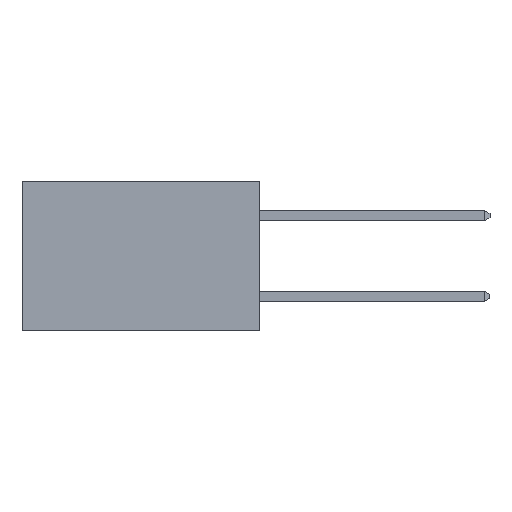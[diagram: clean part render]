
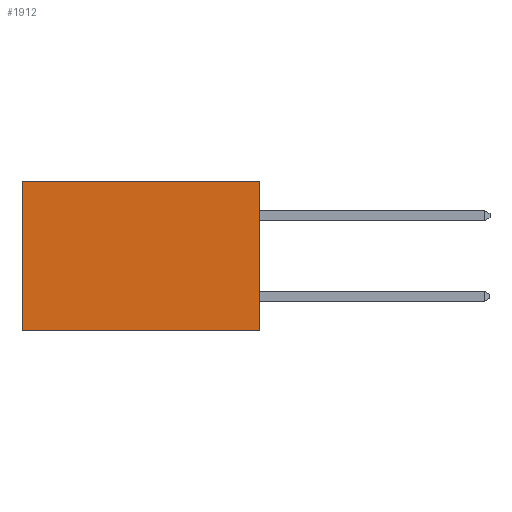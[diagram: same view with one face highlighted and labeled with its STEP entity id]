
A CAD part, left-side view. The second image highlights one B-rep face of the part: STEP entity #1912.
In plain terms, the highlighted planar face has unit normal (-1, 0, 0).
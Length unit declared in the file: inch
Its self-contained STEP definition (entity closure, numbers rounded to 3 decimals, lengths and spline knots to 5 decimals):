
#59 = DIRECTION ( 'NONE',  ( 0., 1., 0. ) ) ;
#163 = DIRECTION ( 'NONE',  ( 0., 1., 0. ) ) ;
#403 = EDGE_LOOP ( 'NONE', ( #11225, #3974, #9107, #4269 ) ) ;
#441 = LINE ( 'NONE', #2921, #5228 ) ;
#537 = EDGE_CURVE ( 'NONE', #11483, #9231, #3000, .T. ) ;
#574 = CARTESIAN_POINT ( 'NONE',  ( 0.277, 0., -0.37 ) ) ;
#1319 = AXIS2_PLACEMENT_3D ( 'NONE', #8702, #7791, #8006 ) ;
#1912 = ADVANCED_FACE ( 'NONE', ( #4821 ), #11175, .F. ) ;
#2921 = CARTESIAN_POINT ( 'NONE',  ( 0.277, 0.59, -0.37 ) ) ;
#3000 = LINE ( 'NONE', #10375, #7812 ) ;
#3184 = CARTESIAN_POINT ( 'NONE',  ( 0.277, 0., 0. ) ) ;
#3367 = EDGE_CURVE ( 'NONE', #11483, #10860, #7313, .T. ) ;
#3582 = CARTESIAN_POINT ( 'NONE',  ( 0.277, 0.59, 0. ) ) ;
#3947 = EDGE_CURVE ( 'NONE', #9231, #10723, #10871, .T. ) ;
#3973 = CARTESIAN_POINT ( 'NONE',  ( 0.277, 0.59, -0.37 ) ) ;
#3974 = ORIENTED_EDGE ( 'NONE', *, *, #3947, .F. ) ;
#4269 = ORIENTED_EDGE ( 'NONE', *, *, #3367, .T. ) ;
#4737 = EDGE_CURVE ( 'NONE', #10860, #10723, #441, .T. ) ;
#4821 = FACE_OUTER_BOUND ( 'NONE', #403, .T. ) ;
#5228 = VECTOR ( 'NONE', #11977, 39.37008 ) ;
#7313 = LINE ( 'NONE', #3184, #11986 ) ;
#7430 = CARTESIAN_POINT ( 'NONE',  ( 0.277, 0., 0. ) ) ;
#7791 = DIRECTION ( 'NONE',  ( 1., 0., 0. ) ) ;
#7812 = VECTOR ( 'NONE', #11929, 39.37008 ) ;
#8006 = DIRECTION ( 'NONE',  ( 0., 0., -1. ) ) ;
#8330 = CARTESIAN_POINT ( 'NONE',  ( 0.277, 0., -0.37 ) ) ;
#8377 = VECTOR ( 'NONE', #163, 39.37008 ) ;
#8702 = CARTESIAN_POINT ( 'NONE',  ( 0.277, 0., -0.37 ) ) ;
#9107 = ORIENTED_EDGE ( 'NONE', *, *, #537, .F. ) ;
#9231 = VERTEX_POINT ( 'NONE', #8330 ) ;
#10375 = CARTESIAN_POINT ( 'NONE',  ( 0.277, 0., -0.37 ) ) ;
#10723 = VERTEX_POINT ( 'NONE', #3973 ) ;
#10860 = VERTEX_POINT ( 'NONE', #3582 ) ;
#10871 = LINE ( 'NONE', #574, #8377 ) ;
#11175 = PLANE ( 'NONE',  #1319 ) ;
#11225 = ORIENTED_EDGE ( 'NONE', *, *, #4737, .T. ) ;
#11483 = VERTEX_POINT ( 'NONE', #7430 ) ;
#11929 = DIRECTION ( 'NONE',  ( 0., 0., -1. ) ) ;
#11977 = DIRECTION ( 'NONE',  ( 0., 0., -1. ) ) ;
#11986 = VECTOR ( 'NONE', #59, 39.37008 ) ;
